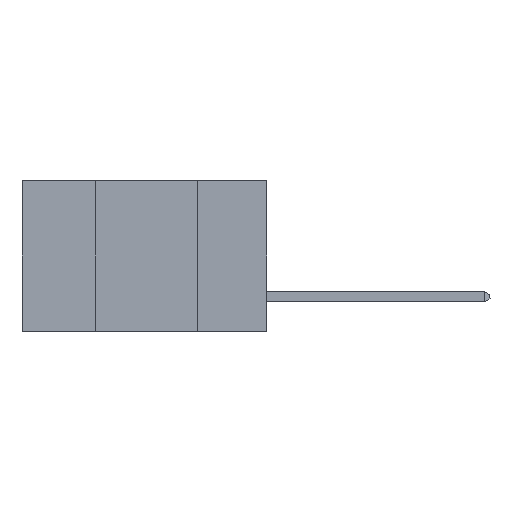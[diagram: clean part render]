
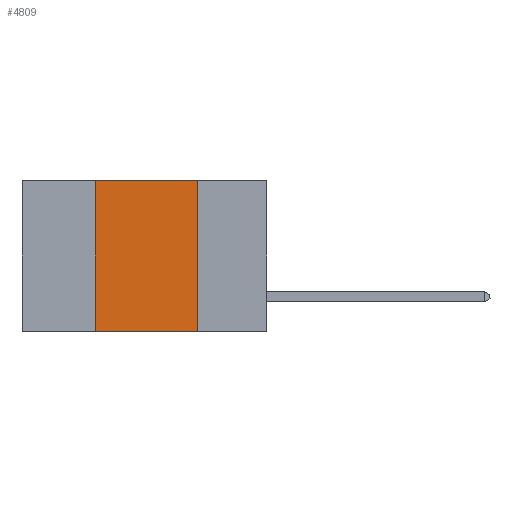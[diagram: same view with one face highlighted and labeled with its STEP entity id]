
A CAD part, left-side view. The second image highlights one B-rep face of the part: STEP entity #4809.
In plain terms, the highlighted planar face has unit normal (-1, 0, 0).
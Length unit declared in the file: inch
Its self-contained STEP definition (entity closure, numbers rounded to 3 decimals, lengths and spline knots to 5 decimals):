
#496 = DIRECTION ( 'NONE',  ( 0., -1., 0. ) ) ;
#1388 = VECTOR ( 'NONE', #496, 39.37008 ) ;
#1739 = VECTOR ( 'NONE', #7958, 39.37008 ) ;
#1756 = LINE ( 'NONE', #7189, #1388 ) ;
#2016 = EDGE_CURVE ( 'NONE', #5972, #6214, #3662, .T. ) ;
#2302 = CARTESIAN_POINT ( 'NONE',  ( 0., 0.42, 0. ) ) ;
#3662 = LINE ( 'NONE', #12203, #1739 ) ;
#4010 = CARTESIAN_POINT ( 'NONE',  ( 0., 0.6, -0.37 ) ) ;
#4809 = ADVANCED_FACE ( 'NONE', ( #10721 ), #5598, .F. ) ;
#4866 = CARTESIAN_POINT ( 'NONE',  ( 0., 0.17, 0. ) ) ;
#4902 = VECTOR ( 'NONE', #10692, 39.37008 ) ;
#5598 = PLANE ( 'NONE',  #7092 ) ;
#5972 = VERTEX_POINT ( 'NONE', #12382 ) ;
#6128 = VERTEX_POINT ( 'NONE', #4866 ) ;
#6214 = VERTEX_POINT ( 'NONE', #2302 ) ;
#6481 = DIRECTION ( 'NONE',  ( 0., 0., -1. ) ) ;
#6572 = DIRECTION ( 'NONE',  ( 1., 0., 0. ) ) ;
#7092 = AXIS2_PLACEMENT_3D ( 'NONE', #12069, #6572, #7836 ) ;
#7189 = CARTESIAN_POINT ( 'NONE',  ( 0., 0.6, 0. ) ) ;
#7268 = ORIENTED_EDGE ( 'NONE', *, *, #2016, .F. ) ;
#7529 = CARTESIAN_POINT ( 'NONE',  ( 0., 0.17, -0.37 ) ) ;
#7602 = ORIENTED_EDGE ( 'NONE', *, *, #11752, .F. ) ;
#7836 = DIRECTION ( 'NONE',  ( 0., 0., -1. ) ) ;
#7958 = DIRECTION ( 'NONE',  ( 0., 0., 1. ) ) ;
#8297 = EDGE_LOOP ( 'NONE', ( #7602, #12142, #7268, #13618 ) ) ;
#9785 = CARTESIAN_POINT ( 'NONE',  ( 0., 0.17, 0. ) ) ;
#10692 = DIRECTION ( 'NONE',  ( 0., -1., 0. ) ) ;
#10721 = FACE_OUTER_BOUND ( 'NONE', #8297, .T. ) ;
#10782 = LINE ( 'NONE', #4010, #4902 ) ;
#11752 = EDGE_CURVE ( 'NONE', #6128, #12497, #12714, .T. ) ;
#12069 = CARTESIAN_POINT ( 'NONE',  ( 0., 0.6, 0. ) ) ;
#12142 = ORIENTED_EDGE ( 'NONE', *, *, #12321, .F. ) ;
#12203 = CARTESIAN_POINT ( 'NONE',  ( 0., 0.42, 0. ) ) ;
#12321 = EDGE_CURVE ( 'NONE', #6214, #6128, #1756, .T. ) ;
#12382 = CARTESIAN_POINT ( 'NONE',  ( 0., 0.42, -0.37 ) ) ;
#12497 = VERTEX_POINT ( 'NONE', #7529 ) ;
#12714 = LINE ( 'NONE', #9785, #13918 ) ;
#12904 = EDGE_CURVE ( 'NONE', #5972, #12497, #10782, .T. ) ;
#13618 = ORIENTED_EDGE ( 'NONE', *, *, #12904, .T. ) ;
#13918 = VECTOR ( 'NONE', #6481, 39.37008 ) ;
